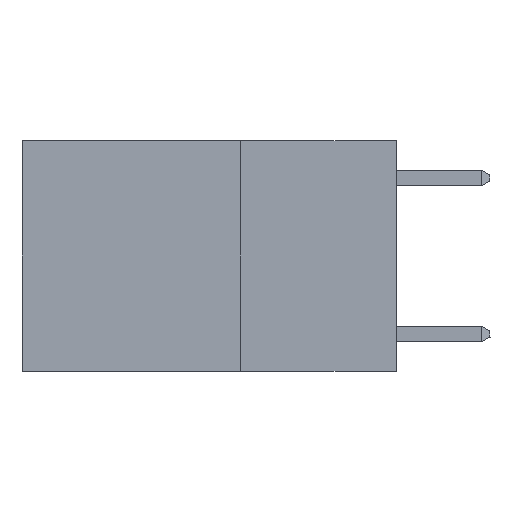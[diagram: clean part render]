
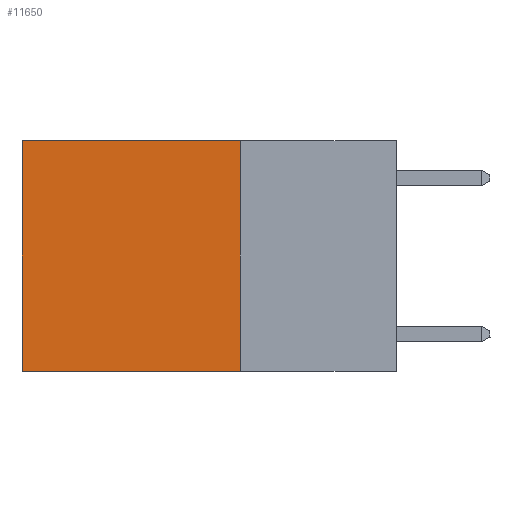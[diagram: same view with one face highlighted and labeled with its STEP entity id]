
A CAD part, left-side view. The second image highlights one B-rep face of the part: STEP entity #11650.
In plain terms, the highlighted planar face has unit normal (-1, 0, 0).
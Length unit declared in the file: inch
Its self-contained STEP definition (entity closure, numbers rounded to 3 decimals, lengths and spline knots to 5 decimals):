
#127 = VERTEX_POINT ( 'NONE', #8653 ) ;
#200 = VECTOR ( 'NONE', #10726, 39.37008 ) ;
#204 = VERTEX_POINT ( 'NONE', #746 ) ;
#288 = CARTESIAN_POINT ( 'NONE',  ( 0.2625, 0.25, -0.37 ) ) ;
#522 = LINE ( 'NONE', #3553, #200 ) ;
#746 = CARTESIAN_POINT ( 'NONE',  ( 0.2625, 0.6, 0. ) ) ;
#763 = LINE ( 'NONE', #11678, #3138 ) ;
#808 = VECTOR ( 'NONE', #1279, 39.37008 ) ;
#864 = VERTEX_POINT ( 'NONE', #6629 ) ;
#1113 = LINE ( 'NONE', #288, #808 ) ;
#1162 = EDGE_CURVE ( 'NONE', #204, #864, #522, .T. ) ;
#1203 = VERTEX_POINT ( 'NONE', #7448 ) ;
#1279 = DIRECTION ( 'NONE',  ( 0., 1., 0. ) ) ;
#1484 = EDGE_CURVE ( 'NONE', #1203, #864, #1113, .T. ) ;
#2086 = ORIENTED_EDGE ( 'NONE', *, *, #1162, .T. ) ;
#2193 = EDGE_CURVE ( 'NONE', #127, #1203, #2329, .T. ) ;
#2329 = LINE ( 'NONE', #5089, #6605 ) ;
#2512 = EDGE_CURVE ( 'NONE', #127, #204, #763, .T. ) ;
#2938 = ORIENTED_EDGE ( 'NONE', *, *, #2512, .T. ) ;
#3138 = VECTOR ( 'NONE', #7572, 39.37008 ) ;
#3513 = EDGE_LOOP ( 'NONE', ( #2086, #7666, #7545, #2938 ) ) ;
#3553 = CARTESIAN_POINT ( 'NONE',  ( 0.2625, 0.6, 0. ) ) ;
#3723 = DIRECTION ( 'NONE',  ( 1., 0., 0. ) ) ;
#4681 = FACE_OUTER_BOUND ( 'NONE', #3513, .T. ) ;
#5089 = CARTESIAN_POINT ( 'NONE',  ( 0.2625, 0.25, 0. ) ) ;
#6605 = VECTOR ( 'NONE', #11075, 39.37008 ) ;
#6629 = CARTESIAN_POINT ( 'NONE',  ( 0.2625, 0.6, -0.37 ) ) ;
#7448 = CARTESIAN_POINT ( 'NONE',  ( 0.2625, 0.25, -0.37 ) ) ;
#7514 = CARTESIAN_POINT ( 'NONE',  ( 0.2625, 0.25, 0. ) ) ;
#7545 = ORIENTED_EDGE ( 'NONE', *, *, #2193, .F. ) ;
#7572 = DIRECTION ( 'NONE',  ( 0., 1., 0. ) ) ;
#7666 = ORIENTED_EDGE ( 'NONE', *, *, #1484, .F. ) ;
#8653 = CARTESIAN_POINT ( 'NONE',  ( 0.2625, 0.25, 0. ) ) ;
#9152 = AXIS2_PLACEMENT_3D ( 'NONE', #7514, #3723, #10101 ) ;
#9251 = PLANE ( 'NONE',  #9152 ) ;
#10101 = DIRECTION ( 'NONE',  ( 0., 0., -1. ) ) ;
#10726 = DIRECTION ( 'NONE',  ( 0., 0., -1. ) ) ;
#11075 = DIRECTION ( 'NONE',  ( 0., 0., -1. ) ) ;
#11650 = ADVANCED_FACE ( 'NONE', ( #4681 ), #9251, .F. ) ;
#11678 = CARTESIAN_POINT ( 'NONE',  ( 0.2625, 0.25, 0. ) ) ;
